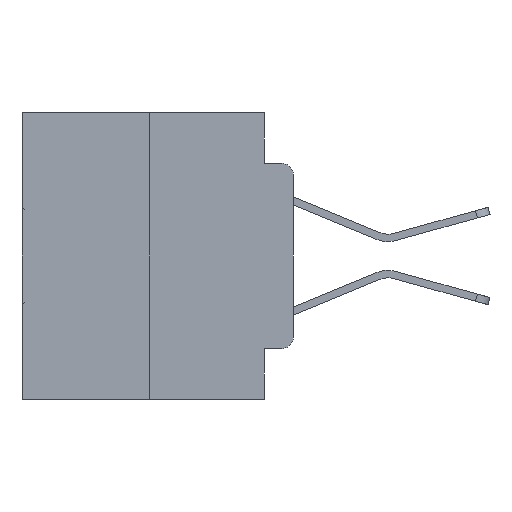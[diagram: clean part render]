
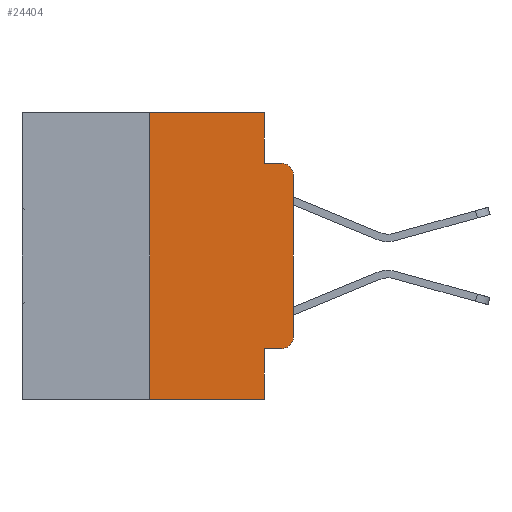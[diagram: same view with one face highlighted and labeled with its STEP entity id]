
A CAD part, left-side view. The second image highlights one B-rep face of the part: STEP entity #24404.
In plain terms, the highlighted planar face has unit normal (-1, 0, 0).
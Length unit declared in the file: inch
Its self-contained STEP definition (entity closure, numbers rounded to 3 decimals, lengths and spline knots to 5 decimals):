
#973 = DIRECTION ( 'NONE',  ( 0., -1., 0. ) ) ;
#1434 = CARTESIAN_POINT ( 'NONE',  ( 0., 0.051, -0.4115 ) ) ;
#2620 = ORIENTED_EDGE ( 'NONE', *, *, #29564, .F. ) ;
#3344 = CARTESIAN_POINT ( 'NONE',  ( 0., 0., 0. ) ) ;
#3460 = CARTESIAN_POINT ( 'NONE',  ( 0., 0.02, -0.3915 ) ) ;
#3615 = CARTESIAN_POINT ( 'NONE',  ( 0., 0.02, -0.0885 ) ) ;
#3789 = DIRECTION ( 'NONE',  ( 0., 0., 1. ) ) ;
#4033 = CARTESIAN_POINT ( 'NONE',  ( 0., 0.051, 0. ) ) ;
#4320 = VERTEX_POINT ( 'NONE', #19722 ) ;
#5294 = CARTESIAN_POINT ( 'NONE',  ( 0., 0.051, -0.5 ) ) ;
#5596 = DIRECTION ( 'NONE',  ( 0., 0., -1. ) ) ;
#6137 = CARTESIAN_POINT ( 'NONE',  ( 0., 0.02, -0.1085 ) ) ;
#6458 = ORIENTED_EDGE ( 'NONE', *, *, #12319, .F. ) ;
#7272 = AXIS2_PLACEMENT_3D ( 'NONE', #3460, #15097, #14951 ) ;
#7429 = VECTOR ( 'NONE', #5596, 39.37008 ) ;
#7645 = VECTOR ( 'NONE', #7772, 39.37008 ) ;
#7772 = DIRECTION ( 'NONE',  ( 0., 0., 1. ) ) ;
#8218 = DIRECTION ( 'NONE',  ( 0., -1., 0. ) ) ;
#8280 = CARTESIAN_POINT ( 'NONE',  ( 0., 0., -0.3915 ) ) ;
#8386 = LINE ( 'NONE', #26460, #20735 ) ;
#8505 = EDGE_CURVE ( 'NONE', #20046, #13027, #11101, .T. ) ;
#9540 = VECTOR ( 'NONE', #26910, 39.37008 ) ;
#9709 = ORIENTED_EDGE ( 'NONE', *, *, #28507, .F. ) ;
#10211 = CARTESIAN_POINT ( 'NONE',  ( 0., 0.02, -0.4115 ) ) ;
#10710 = CARTESIAN_POINT ( 'NONE',  ( 0., 0.25, -0.5 ) ) ;
#10988 = LINE ( 'NONE', #4033, #7429 ) ;
#11101 = LINE ( 'NONE', #22239, #9540 ) ;
#11179 = EDGE_CURVE ( 'NONE', #14522, #16071, #21501, .T. ) ;
#11484 = VERTEX_POINT ( 'NONE', #1434 ) ;
#12107 = VERTEX_POINT ( 'NONE', #5294 ) ;
#12319 = EDGE_CURVE ( 'NONE', #11484, #12107, #10988, .T. ) ;
#12435 = LINE ( 'NONE', #21634, #23997 ) ;
#12569 = VERTEX_POINT ( 'NONE', #10211 ) ;
#12746 = EDGE_CURVE ( 'NONE', #14522, #12107, #8386, .T. ) ;
#13027 = VERTEX_POINT ( 'NONE', #28400 ) ;
#14080 = ORIENTED_EDGE ( 'NONE', *, *, #8505, .F. ) ;
#14319 = FACE_OUTER_BOUND ( 'NONE', #22280, .T. ) ;
#14522 = VERTEX_POINT ( 'NONE', #10710 ) ;
#14743 = CARTESIAN_POINT ( 'NONE',  ( 0., 0.25, 0. ) ) ;
#14912 = EDGE_CURVE ( 'NONE', #4320, #20302, #16040, .T. ) ;
#14951 = DIRECTION ( 'NONE',  ( 0., 0., -1. ) ) ;
#15085 = AXIS2_PLACEMENT_3D ( 'NONE', #6137, #22941, #24505 ) ;
#15097 = DIRECTION ( 'NONE',  ( -1., 0., 0. ) ) ;
#15979 = AXIS2_PLACEMENT_3D ( 'NONE', #16425, #18845, #19004 ) ;
#16006 = CARTESIAN_POINT ( 'NONE',  ( 0., 0.473, 0. ) ) ;
#16040 = CIRCLE ( 'NONE', #15085, 0.02 ) ;
#16071 = VERTEX_POINT ( 'NONE', #27690 ) ;
#16425 = CARTESIAN_POINT ( 'NONE',  ( 0., 0.473, 0. ) ) ;
#16605 = ORIENTED_EDGE ( 'NONE', *, *, #24047, .T. ) ;
#17139 = CARTESIAN_POINT ( 'NONE',  ( 0., 0.051, -0.0885 ) ) ;
#17589 = DIRECTION ( 'NONE',  ( 0., -1., 0. ) ) ;
#17683 = ORIENTED_EDGE ( 'NONE', *, *, #12746, .T. ) ;
#18419 = DIRECTION ( 'NONE',  ( 0., -1., 0. ) ) ;
#18535 = PLANE ( 'NONE',  #15979 ) ;
#18577 = EDGE_CURVE ( 'NONE', #26063, #4320, #23977, .T. ) ;
#18845 = DIRECTION ( 'NONE',  ( 1., 0., 0. ) ) ;
#19004 = DIRECTION ( 'NONE',  ( 0., 0., -1. ) ) ;
#19637 = ORIENTED_EDGE ( 'NONE', *, *, #11179, .F. ) ;
#19722 = CARTESIAN_POINT ( 'NONE',  ( 0., 0., -0.1085 ) ) ;
#19900 = EDGE_CURVE ( 'NONE', #11484, #12569, #12435, .T. ) ;
#20004 = ORIENTED_EDGE ( 'NONE', *, *, #19900, .T. ) ;
#20037 = ORIENTED_EDGE ( 'NONE', *, *, #14912, .T. ) ;
#20046 = VERTEX_POINT ( 'NONE', #25050 ) ;
#20302 = VERTEX_POINT ( 'NONE', #3615 ) ;
#20512 = VECTOR ( 'NONE', #18419, 39.37008 ) ;
#20735 = VECTOR ( 'NONE', #17589, 39.37008 ) ;
#21094 = VECTOR ( 'NONE', #3789, 39.37008 ) ;
#21501 = LINE ( 'NONE', #14743, #7645 ) ;
#21634 = CARTESIAN_POINT ( 'NONE',  ( 0., 0.051, -0.4115 ) ) ;
#21743 = CIRCLE ( 'NONE', #7272, 0.02 ) ;
#22239 = CARTESIAN_POINT ( 'NONE',  ( 0., 0.051, 0. ) ) ;
#22280 = EDGE_LOOP ( 'NONE', ( #22905, #20037, #2620, #14080, #9709, #19637, #17683, #6458, #20004, #16605 ) ) ;
#22905 = ORIENTED_EDGE ( 'NONE', *, *, #18577, .T. ) ;
#22941 = DIRECTION ( 'NONE',  ( -1., 0., 0. ) ) ;
#23332 = VECTOR ( 'NONE', #8218, 39.37008 ) ;
#23977 = LINE ( 'NONE', #3344, #21094 ) ;
#23997 = VECTOR ( 'NONE', #973, 39.37008 ) ;
#24047 = EDGE_CURVE ( 'NONE', #12569, #26063, #21743, .T. ) ;
#24404 = ADVANCED_FACE ( 'NONE', ( #14319 ), #18535, .F. ) ;
#24505 = DIRECTION ( 'NONE',  ( 0., 0., -1. ) ) ;
#24873 = LINE ( 'NONE', #16006, #20512 ) ;
#25050 = CARTESIAN_POINT ( 'NONE',  ( 0., 0.051, 0. ) ) ;
#26063 = VERTEX_POINT ( 'NONE', #8280 ) ;
#26303 = LINE ( 'NONE', #17139, #23332 ) ;
#26460 = CARTESIAN_POINT ( 'NONE',  ( 0., 0.473, -0.5 ) ) ;
#26910 = DIRECTION ( 'NONE',  ( 0., 0., -1. ) ) ;
#27690 = CARTESIAN_POINT ( 'NONE',  ( 0., 0.25, 0. ) ) ;
#28400 = CARTESIAN_POINT ( 'NONE',  ( 0., 0.051, -0.0885 ) ) ;
#28507 = EDGE_CURVE ( 'NONE', #16071, #20046, #24873, .T. ) ;
#29564 = EDGE_CURVE ( 'NONE', #13027, #20302, #26303, .T. ) ;
